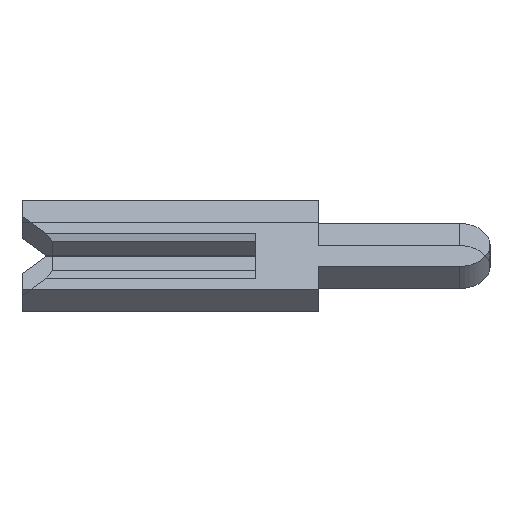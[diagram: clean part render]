
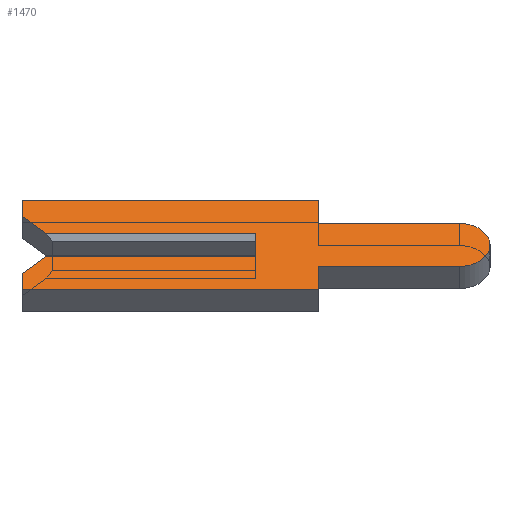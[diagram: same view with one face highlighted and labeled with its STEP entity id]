
A CAD part, left-side view. The second image highlights one B-rep face of the part: STEP entity #1470.
In plain terms, the highlighted face is planar.
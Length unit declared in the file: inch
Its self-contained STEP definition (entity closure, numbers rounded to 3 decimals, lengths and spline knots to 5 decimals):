
#1 = CARTESIAN_POINT ( 'NONE',  ( -0.01, 0.134, 0.01 ) ) ;
#15 = DIRECTION ( 'NONE',  ( 0., 0., 1. ) ) ;
#57 = CARTESIAN_POINT ( 'NONE',  ( -0.01, 0.15, -0.04 ) ) ;
#122 = VERTEX_POINT ( 'NONE', #1382 ) ;
#190 = VECTOR ( 'NONE', #1443, 39.37008 ) ;
#228 = LINE ( 'NONE', #2560, #2353 ) ;
#256 = CARTESIAN_POINT ( 'NONE',  ( -0.01, -0.04, -0.0195 ) ) ;
#261 = VECTOR ( 'NONE', #1388, 39.37008 ) ;
#271 = VECTOR ( 'NONE', #15, 39.37008 ) ;
#367 = LINE ( 'NONE', #3406, #3289 ) ;
#400 = CARTESIAN_POINT ( 'NONE',  ( -0.01, 0.15, 0.04 ) ) ;
#426 = DIRECTION ( 'NONE',  ( 0., 0., -1. ) ) ;
#491 = EDGE_CURVE ( 'NONE', #824, #2844, #228, .T. ) ;
#492 = VECTOR ( 'NONE', #3568, 39.37008 ) ;
#505 = CARTESIAN_POINT ( 'NONE',  ( -0.01, -0.04, -0.04 ) ) ;
#540 = EDGE_CURVE ( 'NONE', #1171, #873, #3023, .T. ) ;
#558 = DIRECTION ( 'NONE',  ( 0., -1., 0. ) ) ;
#591 = EDGE_CURVE ( 'NONE', #1036, #2205, #3413, .T. ) ;
#665 = DIRECTION ( 'NONE',  ( 0., -1., 0. ) ) ;
#703 = CARTESIAN_POINT ( 'NONE',  ( -0.01, -0.04, 0.04 ) ) ;
#708 = LINE ( 'NONE', #1611, #492 ) ;
#760 = CARTESIAN_POINT ( 'NONE',  ( -0.01, -0.04, 0.0195 ) ) ;
#782 = EDGE_CURVE ( 'NONE', #2895, #2844, #367, .T. ) ;
#793 = CARTESIAN_POINT ( 'NONE',  ( -0.01, -0.04, -0.0195 ) ) ;
#820 = ORIENTED_EDGE ( 'NONE', *, *, #1315, .F. ) ;
#824 = VERTEX_POINT ( 'NONE', #1 ) ;
#850 = EDGE_CURVE ( 'NONE', #873, #2424, #936, .T. ) ;
#873 = VERTEX_POINT ( 'NONE', #3095 ) ;
#895 = AXIS2_PLACEMENT_3D ( 'NONE', #3178, #2909, #2013 ) ;
#936 = LINE ( 'NONE', #1167, #190 ) ;
#947 = CARTESIAN_POINT ( 'NONE',  ( -0.01, -0.1305, 0. ) ) ;
#980 = ORIENTED_EDGE ( 'NONE', *, *, #850, .F. ) ;
#1014 = LINE ( 'NONE', #793, #261 ) ;
#1017 = LINE ( 'NONE', #760, #1792 ) ;
#1036 = VERTEX_POINT ( 'NONE', #2305 ) ;
#1050 = DIRECTION ( 'NONE',  ( 0., -1., 0. ) ) ;
#1098 = CARTESIAN_POINT ( 'NONE',  ( -0.01, -0.04, 0.0195 ) ) ;
#1167 = CARTESIAN_POINT ( 'NONE',  ( -0.01, 0.1305, -0.0065 ) ) ;
#1171 = VERTEX_POINT ( 'NONE', #57 ) ;
#1187 = ORIENTED_EDGE ( 'NONE', *, *, #2618, .F. ) ;
#1188 = ORIENTED_EDGE ( 'NONE', *, *, #2435, .F. ) ;
#1269 = DIRECTION ( 'NONE',  ( 1., 0., 0. ) ) ;
#1315 = EDGE_CURVE ( 'NONE', #824, #1036, #1583, .T. ) ;
#1382 = CARTESIAN_POINT ( 'NONE',  ( -0.01, -0.1305, -0.0195 ) ) ;
#1388 = DIRECTION ( 'NONE',  ( 0., 1., 0. ) ) ;
#1408 = DIRECTION ( 'NONE',  ( 0., 0., 1. ) ) ;
#1443 = DIRECTION ( 'NONE',  ( 0., -0.707, 0.707 ) ) ;
#1470 = ADVANCED_FACE ( 'NONE', ( #2987 ), #1502, .F. ) ;
#1493 = ORIENTED_EDGE ( 'NONE', *, *, #591, .F. ) ;
#1502 = PLANE ( 'NONE',  #895 ) ;
#1554 = DIRECTION ( 'NONE',  ( 0., 0., -1. ) ) ;
#1583 = LINE ( 'NONE', #2292, #2155 ) ;
#1611 = CARTESIAN_POINT ( 'NONE',  ( -0.01, -0.1305, -0.01 ) ) ;
#1625 = CARTESIAN_POINT ( 'NONE',  ( -0.01, 0., 0.01 ) ) ;
#1650 = ORIENTED_EDGE ( 'NONE', *, *, #2058, .F. ) ;
#1676 = DIRECTION ( 'NONE',  ( 0., 0., 1. ) ) ;
#1681 = VECTOR ( 'NONE', #2766, 39.37008 ) ;
#1732 = EDGE_CURVE ( 'NONE', #2205, #1936, #3221, .T. ) ;
#1792 = VECTOR ( 'NONE', #1050, 39.37008 ) ;
#1881 = ORIENTED_EDGE ( 'NONE', *, *, #1732, .F. ) ;
#1900 = AXIS2_PLACEMENT_3D ( 'NONE', #947, #1269, #1554 ) ;
#1936 = VERTEX_POINT ( 'NONE', #703 ) ;
#2013 = DIRECTION ( 'NONE',  ( 0., 0., -1. ) ) ;
#2021 = VERTEX_POINT ( 'NONE', #3496 ) ;
#2058 = EDGE_CURVE ( 'NONE', #2904, #122, #3237, .T. ) ;
#2071 = ORIENTED_EDGE ( 'NONE', *, *, #491, .T. ) ;
#2076 = CARTESIAN_POINT ( 'NONE',  ( -0.01, 0.15, -0.04 ) ) ;
#2112 = ORIENTED_EDGE ( 'NONE', *, *, #3402, .F. ) ;
#2154 = ORIENTED_EDGE ( 'NONE', *, *, #540, .F. ) ;
#2155 = VECTOR ( 'NONE', #3201, 39.37008 ) ;
#2156 = ORIENTED_EDGE ( 'NONE', *, *, #2255, .F. ) ;
#2160 = EDGE_CURVE ( 'NONE', #2021, #1171, #2384, .T. ) ;
#2176 = CARTESIAN_POINT ( 'NONE',  ( -0.01, 0.134, -0.01 ) ) ;
#2205 = VERTEX_POINT ( 'NONE', #3522 ) ;
#2221 = LINE ( 'NONE', #3505, #3279 ) ;
#2255 = EDGE_CURVE ( 'NONE', #1936, #3176, #2221, .T. ) ;
#2271 = VECTOR ( 'NONE', #1676, 39.37008 ) ;
#2292 = CARTESIAN_POINT ( 'NONE',  ( -0.01, 0.1305, 0.0065 ) ) ;
#2305 = CARTESIAN_POINT ( 'NONE',  ( -0.01, 0.15, 0.026 ) ) ;
#2315 = VECTOR ( 'NONE', #665, 39.37008 ) ;
#2334 = EDGE_LOOP ( 'NONE', ( #2071, #3303, #1188, #980, #2154, #2673, #2112, #2813, #1650, #1187, #2156, #1881, #1493, #820 ) ) ;
#2353 = VECTOR ( 'NONE', #558, 39.37008 ) ;
#2384 = LINE ( 'NONE', #2076, #2968 ) ;
#2424 = VERTEX_POINT ( 'NONE', #2176 ) ;
#2435 = EDGE_CURVE ( 'NONE', #2424, #2895, #708, .T. ) ;
#2560 = CARTESIAN_POINT ( 'NONE',  ( -0.01, 0.15, 0.01 ) ) ;
#2601 = LINE ( 'NONE', #505, #1681 ) ;
#2618 = EDGE_CURVE ( 'NONE', #3176, #2904, #1017, .T. ) ;
#2673 = ORIENTED_EDGE ( 'NONE', *, *, #2160, .F. ) ;
#2678 = DIRECTION ( 'NONE',  ( 0., 1., 0. ) ) ;
#2749 = CARTESIAN_POINT ( 'NONE',  ( -0.01, -0.1305, 0.0195 ) ) ;
#2766 = DIRECTION ( 'NONE',  ( 0., 0., -1. ) ) ;
#2813 = ORIENTED_EDGE ( 'NONE', *, *, #3388, .F. ) ;
#2822 = CARTESIAN_POINT ( 'NONE',  ( -0.01, 0.15, 0.026 ) ) ;
#2842 = CARTESIAN_POINT ( 'NONE',  ( -0.01, 0.15, -0.026 ) ) ;
#2844 = VERTEX_POINT ( 'NONE', #1625 ) ;
#2895 = VERTEX_POINT ( 'NONE', #2992 ) ;
#2904 = VERTEX_POINT ( 'NONE', #2749 ) ;
#2909 = DIRECTION ( 'NONE',  ( 1., 0., 0. ) ) ;
#2968 = VECTOR ( 'NONE', #2678, 39.37008 ) ;
#2987 = FACE_OUTER_BOUND ( 'NONE', #2334, .T. ) ;
#2992 = CARTESIAN_POINT ( 'NONE',  ( -0.01, 0., -0.01 ) ) ;
#3003 = VERTEX_POINT ( 'NONE', #256 ) ;
#3023 = LINE ( 'NONE', #2842, #2271 ) ;
#3095 = CARTESIAN_POINT ( 'NONE',  ( -0.01, 0.15, -0.026 ) ) ;
#3176 = VERTEX_POINT ( 'NONE', #1098 ) ;
#3178 = CARTESIAN_POINT ( 'NONE',  ( -0.01, -0.1305, 0. ) ) ;
#3201 = DIRECTION ( 'NONE',  ( 0., 0.707, 0.707 ) ) ;
#3221 = LINE ( 'NONE', #400, #2315 ) ;
#3237 = CIRCLE ( 'NONE', #1900, 0.0195 ) ;
#3279 = VECTOR ( 'NONE', #426, 39.37008 ) ;
#3289 = VECTOR ( 'NONE', #1408, 39.37008 ) ;
#3303 = ORIENTED_EDGE ( 'NONE', *, *, #782, .F. ) ;
#3388 = EDGE_CURVE ( 'NONE', #122, #3003, #1014, .T. ) ;
#3402 = EDGE_CURVE ( 'NONE', #3003, #2021, #2601, .T. ) ;
#3406 = CARTESIAN_POINT ( 'NONE',  ( -0.01, 0., 0.0065 ) ) ;
#3413 = LINE ( 'NONE', #2822, #271 ) ;
#3496 = CARTESIAN_POINT ( 'NONE',  ( -0.01, -0.04, -0.04 ) ) ;
#3505 = CARTESIAN_POINT ( 'NONE',  ( -0.01, -0.04, 0.04 ) ) ;
#3522 = CARTESIAN_POINT ( 'NONE',  ( -0.01, 0.15, 0.04 ) ) ;
#3568 = DIRECTION ( 'NONE',  ( 0., -1., 0. ) ) ;
